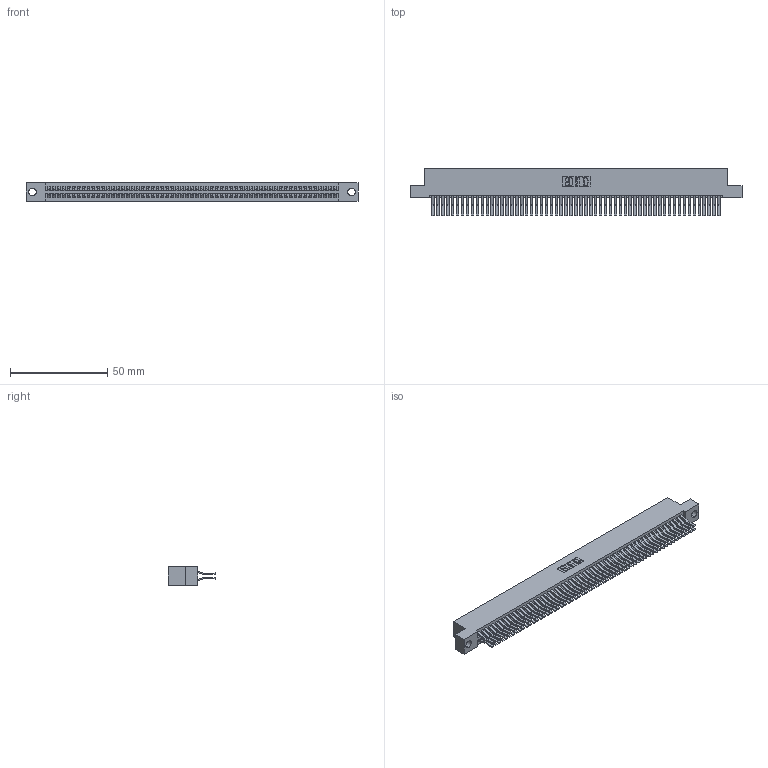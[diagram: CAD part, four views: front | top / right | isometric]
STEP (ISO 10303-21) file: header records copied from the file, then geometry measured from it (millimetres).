
FILE_DESCRIPTION (( 'STEP AP203' ), '1' );
FILE_NAME ('395-118-560-204.STEP', '2021-06-17T20:28:34', ( '' ), ( '' ), 'SwSTEP 2.0', 'SolidWorks 2020', '' );
FILE_SCHEMA (( 'CONFIG_CONTROL_DESIGN' ));
Length unit declared in the file: inch
Products named in the file (3): 395-118-560-204; 345-292-001_560 Tail; 345 Part_Flush Mounting Lugs - 0.156 Dia-TI
Assembly tree (119 placements, depth 2):
  395-118-560-204
    345 Part_Flush Mounting Lugs - 0.156 Dia-TI
    345-292-001_560 Tail  x118
Bounding box: 171.07 x 24.45 x 9.4 mm (x, y, z)
Volume: 17443.1 mm3; surface area: 27953.9 mm2
Topology: 119 solids, 119 shells, 6276 faces, 18667 edges, 12286 vertices
Faces by surface type: plane 3988, cylinder 2288
Entity records: 44511 total; most frequent: CARTESIAN_POINT 7450, ORIENTED_EDGE 7382, DIRECTION 6551, EDGE_CURVE 3691, LINE 3319, VECTOR 3319, VERTEX_POINT 2458, AXIS2_PLACEMENT_3D 1616
